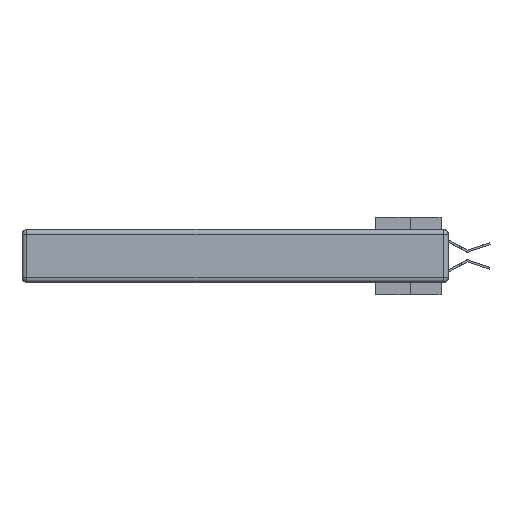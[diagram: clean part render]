
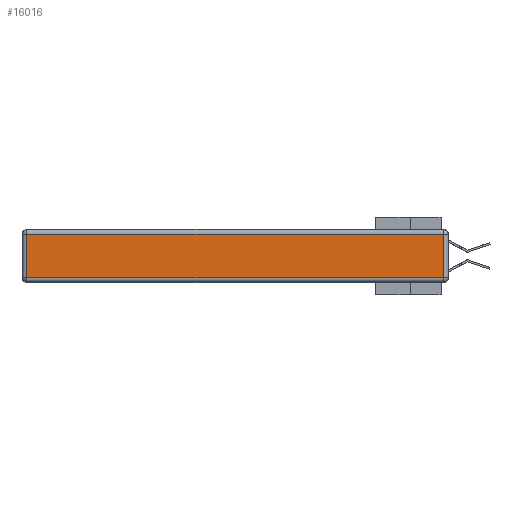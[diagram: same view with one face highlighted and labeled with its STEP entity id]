
A CAD part, left-side view. The second image highlights one B-rep face of the part: STEP entity #16016.
In plain terms, the highlighted planar face has unit normal (-1, 0, 0).
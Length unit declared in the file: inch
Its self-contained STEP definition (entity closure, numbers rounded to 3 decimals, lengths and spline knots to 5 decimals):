
#374 = VECTOR ( 'NONE', #2482, 39.37008 ) ;
#2482 = DIRECTION ( 'NONE',  ( 0., 1., 0. ) ) ;
#2525 = VECTOR ( 'NONE', #17948, 39.37008 ) ;
#3042 = VECTOR ( 'NONE', #30197, 39.37008 ) ;
#4095 = DIRECTION ( 'NONE',  ( 0., -1., 0. ) ) ;
#4148 = CARTESIAN_POINT ( 'NONE',  ( 0., 0.03, -0.313 ) ) ;
#4202 = LINE ( 'NONE', #28668, #2525 ) ;
#4536 = EDGE_CURVE ( 'NONE', #33436, #19856, #4202, .T. ) ;
#5123 = CARTESIAN_POINT ( 'NONE',  ( 0., 2.72, -0.03 ) ) ;
#6655 = EDGE_LOOP ( 'NONE', ( #7945, #31321, #9482, #10851 ) ) ;
#7945 = ORIENTED_EDGE ( 'NONE', *, *, #19368, .T. ) ;
#9482 = ORIENTED_EDGE ( 'NONE', *, *, #18240, .T. ) ;
#10851 = ORIENTED_EDGE ( 'NONE', *, *, #4536, .T. ) ;
#12266 = LINE ( 'NONE', #25297, #3042 ) ;
#12576 = CARTESIAN_POINT ( 'NONE',  ( 0., 0.03, -0.03 ) ) ;
#14243 = CARTESIAN_POINT ( 'NONE',  ( 0., 2.72, -0.313 ) ) ;
#16016 = ADVANCED_FACE ( 'NONE', ( #25187 ), #22742, .T. ) ;
#17638 = CARTESIAN_POINT ( 'NONE',  ( 0., 0., -0.343 ) ) ;
#17948 = DIRECTION ( 'NONE',  ( 0., 0., -1. ) ) ;
#18240 = EDGE_CURVE ( 'NONE', #25678, #33436, #34187, .T. ) ;
#19342 = VECTOR ( 'NONE', #4095, 39.37008 ) ;
#19368 = EDGE_CURVE ( 'NONE', #19856, #25285, #25173, .T. ) ;
#19856 = VERTEX_POINT ( 'NONE', #14243 ) ;
#19919 = EDGE_CURVE ( 'NONE', #25285, #25678, #12266, .T. ) ;
#20073 = CARTESIAN_POINT ( 'NONE',  ( 0., 0., -0.313 ) ) ;
#22620 = AXIS2_PLACEMENT_3D ( 'NONE', #17638, #30912, #28339 ) ;
#22742 = PLANE ( 'NONE',  #22620 ) ;
#23940 = CARTESIAN_POINT ( 'NONE',  ( 0., 2.75, -0.03 ) ) ;
#25173 = LINE ( 'NONE', #20073, #19342 ) ;
#25187 = FACE_OUTER_BOUND ( 'NONE', #6655, .T. ) ;
#25285 = VERTEX_POINT ( 'NONE', #4148 ) ;
#25297 = CARTESIAN_POINT ( 'NONE',  ( 0., 0.03, -0.343 ) ) ;
#25678 = VERTEX_POINT ( 'NONE', #12576 ) ;
#28339 = DIRECTION ( 'NONE',  ( 0., 0., 1. ) ) ;
#28668 = CARTESIAN_POINT ( 'NONE',  ( 0., 2.72, -0.343 ) ) ;
#30197 = DIRECTION ( 'NONE',  ( 0., 0., 1. ) ) ;
#30912 = DIRECTION ( 'NONE',  ( -1., 0., 0. ) ) ;
#31321 = ORIENTED_EDGE ( 'NONE', *, *, #19919, .T. ) ;
#33436 = VERTEX_POINT ( 'NONE', #5123 ) ;
#34187 = LINE ( 'NONE', #23940, #374 ) ;
